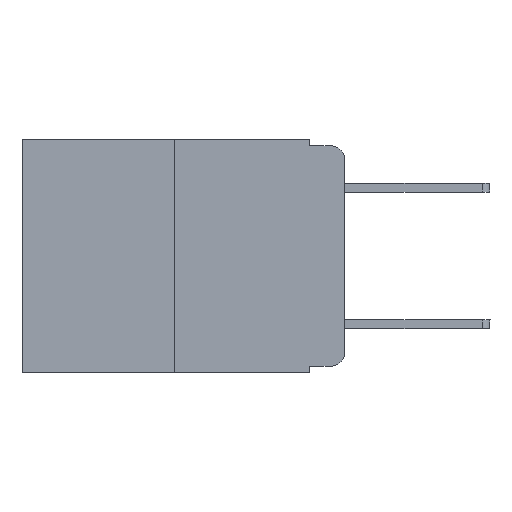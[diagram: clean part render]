
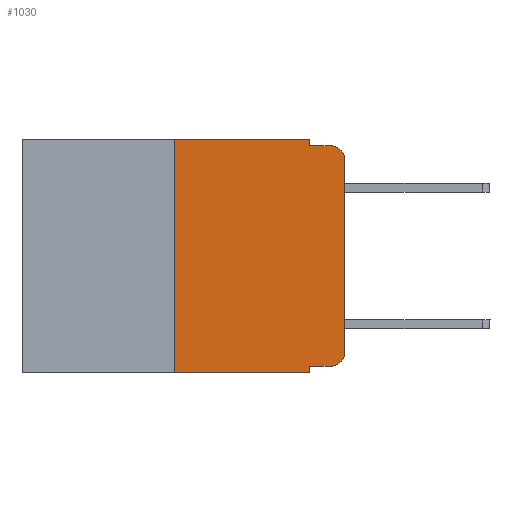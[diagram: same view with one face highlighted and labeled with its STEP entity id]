
A CAD part, left-side view. The second image highlights one B-rep face of the part: STEP entity #1030.
In plain terms, the highlighted planar face has unit normal (-1, 0, 0).
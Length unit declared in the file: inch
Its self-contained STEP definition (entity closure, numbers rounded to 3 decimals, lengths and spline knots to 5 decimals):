
#46 = ORIENTED_EDGE ( 'NONE', *, *, #2297, .F. ) ;
#330 = LINE ( 'NONE', #5017, #1607 ) ;
#556 = CARTESIAN_POINT ( 'NONE',  ( 0., 0.051, -0.01 ) ) ;
#705 = EDGE_CURVE ( 'NONE', #1980, #6303, #885, .T. ) ;
#750 = VERTEX_POINT ( 'NONE', #1257 ) ;
#834 = VERTEX_POINT ( 'NONE', #6880 ) ;
#885 = LINE ( 'NONE', #6697, #4062 ) ;
#1030 = ADVANCED_FACE ( 'NONE', ( #10527 ), #10464, .F. ) ;
#1032 = AXIS2_PLACEMENT_3D ( 'NONE', #9316, #10311, #4311 ) ;
#1257 = CARTESIAN_POINT ( 'NONE',  ( 0., 0.02, -0.333 ) ) ;
#1434 = CIRCLE ( 'NONE', #1032, 0.02 ) ;
#1502 = CARTESIAN_POINT ( 'NONE',  ( 0., 0.051, 0. ) ) ;
#1607 = VECTOR ( 'NONE', #10873, 39.37008 ) ;
#1779 = EDGE_CURVE ( 'NONE', #7100, #750, #5444, .T. ) ;
#1841 = CARTESIAN_POINT ( 'NONE',  ( 0., 0., -0.313 ) ) ;
#1980 = VERTEX_POINT ( 'NONE', #1841 ) ;
#1997 = ORIENTED_EDGE ( 'NONE', *, *, #7398, .T. ) ;
#2119 = VERTEX_POINT ( 'NONE', #10906 ) ;
#2297 = EDGE_CURVE ( 'NONE', #834, #4312, #12110, .T. ) ;
#2433 = ORIENTED_EDGE ( 'NONE', *, *, #705, .T. ) ;
#2650 = CARTESIAN_POINT ( 'NONE',  ( 0., 0.25, 0. ) ) ;
#2905 = CARTESIAN_POINT ( 'NONE',  ( 0., 0.02, -0.01 ) ) ;
#3051 = ORIENTED_EDGE ( 'NONE', *, *, #11035, .F. ) ;
#3229 = VECTOR ( 'NONE', #9982, 39.37008 ) ;
#3463 = VERTEX_POINT ( 'NONE', #2650 ) ;
#3652 = ORIENTED_EDGE ( 'NONE', *, *, #10896, .T. ) ;
#3774 = CARTESIAN_POINT ( 'NONE',  ( 0., 0.473, 0. ) ) ;
#3860 = DIRECTION ( 'NONE',  ( 0., 0., 1. ) ) ;
#3889 = CARTESIAN_POINT ( 'NONE',  ( 0., 0.051, -0.333 ) ) ;
#3891 = DIRECTION ( 'NONE',  ( 0., -1., 0. ) ) ;
#4062 = VECTOR ( 'NONE', #3860, 39.37008 ) ;
#4174 = EDGE_LOOP ( 'NONE', ( #2433, #1997, #46, #6328, #3051, #10225, #6319, #7325, #8038, #3652 ) ) ;
#4311 = DIRECTION ( 'NONE',  ( 0., 0., -1. ) ) ;
#4312 = VERTEX_POINT ( 'NONE', #2905 ) ;
#4550 = AXIS2_PLACEMENT_3D ( 'NONE', #6561, #9532, #11468 ) ;
#4933 = VECTOR ( 'NONE', #9089, 39.37008 ) ;
#5017 = CARTESIAN_POINT ( 'NONE',  ( 0., 0.25, 0. ) ) ;
#5444 = LINE ( 'NONE', #7456, #7537 ) ;
#5599 = DIRECTION ( 'NONE',  ( -1., 0., 0. ) ) ;
#5911 = EDGE_CURVE ( 'NONE', #6720, #3463, #330, .T. ) ;
#6112 = VECTOR ( 'NONE', #3891, 39.37008 ) ;
#6303 = VERTEX_POINT ( 'NONE', #10797 ) ;
#6319 = ORIENTED_EDGE ( 'NONE', *, *, #8238, .T. ) ;
#6328 = ORIENTED_EDGE ( 'NONE', *, *, #12132, .F. ) ;
#6561 = CARTESIAN_POINT ( 'NONE',  ( 0., 0.473, 0. ) ) ;
#6697 = CARTESIAN_POINT ( 'NONE',  ( 0., 0., 0. ) ) ;
#6720 = VERTEX_POINT ( 'NONE', #10524 ) ;
#6880 = CARTESIAN_POINT ( 'NONE',  ( 0., 0.051, -0.01 ) ) ;
#6919 = AXIS2_PLACEMENT_3D ( 'NONE', #12089, #5599, #9457 ) ;
#7100 = VERTEX_POINT ( 'NONE', #3889 ) ;
#7268 = DIRECTION ( 'NONE',  ( 0., -1., 0. ) ) ;
#7318 = LINE ( 'NONE', #12109, #4933 ) ;
#7325 = ORIENTED_EDGE ( 'NONE', *, *, #9099, .F. ) ;
#7398 = EDGE_CURVE ( 'NONE', #6303, #4312, #1434, .T. ) ;
#7453 = CARTESIAN_POINT ( 'NONE',  ( 0., 0.051, -0.343 ) ) ;
#7456 = CARTESIAN_POINT ( 'NONE',  ( 0., 0.051, -0.333 ) ) ;
#7537 = VECTOR ( 'NONE', #7268, 39.37008 ) ;
#7972 = VERTEX_POINT ( 'NONE', #7453 ) ;
#8038 = ORIENTED_EDGE ( 'NONE', *, *, #1779, .T. ) ;
#8140 = CARTESIAN_POINT ( 'NONE',  ( 0., 0.473, -0.343 ) ) ;
#8238 = EDGE_CURVE ( 'NONE', #6720, #7972, #10096, .T. ) ;
#8574 = LINE ( 'NONE', #3774, #6112 ) ;
#9089 = DIRECTION ( 'NONE',  ( 0., 0., -1. ) ) ;
#9099 = EDGE_CURVE ( 'NONE', #7100, #7972, #12290, .T. ) ;
#9284 = VECTOR ( 'NONE', #11227, 39.37008 ) ;
#9316 = CARTESIAN_POINT ( 'NONE',  ( 0., 0.02, -0.03 ) ) ;
#9457 = DIRECTION ( 'NONE',  ( 0., 0., -1. ) ) ;
#9532 = DIRECTION ( 'NONE',  ( 1., 0., 0. ) ) ;
#9982 = DIRECTION ( 'NONE',  ( 0., -1., 0. ) ) ;
#10096 = LINE ( 'NONE', #8140, #3229 ) ;
#10225 = ORIENTED_EDGE ( 'NONE', *, *, #5911, .F. ) ;
#10311 = DIRECTION ( 'NONE',  ( -1., 0., 0. ) ) ;
#10464 = PLANE ( 'NONE',  #4550 ) ;
#10524 = CARTESIAN_POINT ( 'NONE',  ( 0., 0.25, -0.343 ) ) ;
#10527 = FACE_OUTER_BOUND ( 'NONE', #4174, .T. ) ;
#10797 = CARTESIAN_POINT ( 'NONE',  ( 0., 0., -0.03 ) ) ;
#10873 = DIRECTION ( 'NONE',  ( 0., 0., 1. ) ) ;
#10896 = EDGE_CURVE ( 'NONE', #750, #1980, #10931, .T. ) ;
#10906 = CARTESIAN_POINT ( 'NONE',  ( 0., 0.051, 0. ) ) ;
#10931 = CIRCLE ( 'NONE', #6919, 0.02 ) ;
#11035 = EDGE_CURVE ( 'NONE', #3463, #2119, #8574, .T. ) ;
#11227 = DIRECTION ( 'NONE',  ( 0., -1., 0. ) ) ;
#11343 = DIRECTION ( 'NONE',  ( 0., 0., -1. ) ) ;
#11468 = DIRECTION ( 'NONE',  ( 0., 0., -1. ) ) ;
#12089 = CARTESIAN_POINT ( 'NONE',  ( 0., 0.02, -0.313 ) ) ;
#12109 = CARTESIAN_POINT ( 'NONE',  ( 0., 0.051, 0. ) ) ;
#12110 = LINE ( 'NONE', #556, #9284 ) ;
#12112 = VECTOR ( 'NONE', #11343, 39.37008 ) ;
#12132 = EDGE_CURVE ( 'NONE', #2119, #834, #7318, .T. ) ;
#12290 = LINE ( 'NONE', #1502, #12112 ) ;
